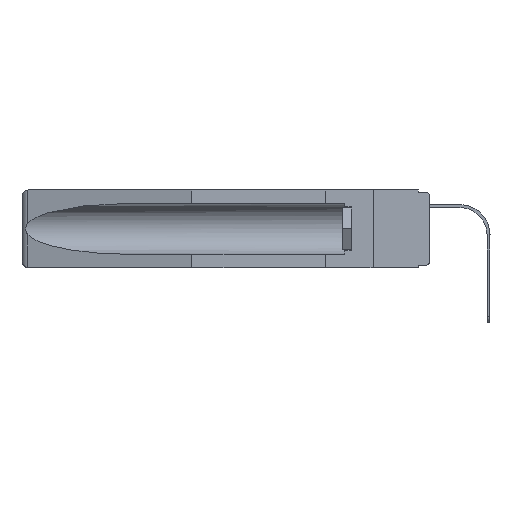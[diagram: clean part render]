
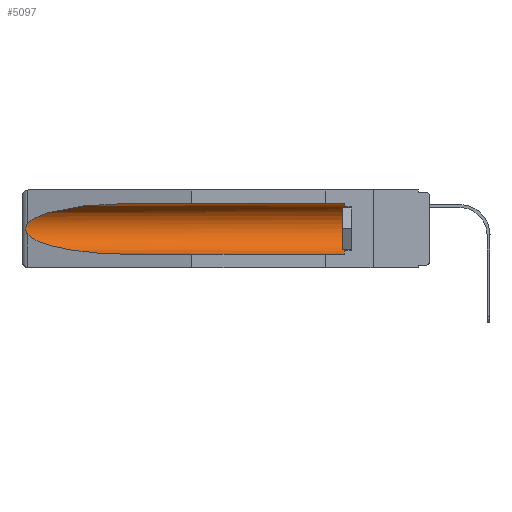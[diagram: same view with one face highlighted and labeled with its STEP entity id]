
A CAD part, left-side view. The second image highlights one B-rep face of the part: STEP entity #5097.
In plain terms, the highlighted cylindrical face has radius 2.857 mm (diameter 5.715 mm), a partial arc.
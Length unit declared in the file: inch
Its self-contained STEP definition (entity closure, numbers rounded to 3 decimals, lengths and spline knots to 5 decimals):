
#67 = DIRECTION ( 'NONE',  ( 0., 1., 0. ) ) ;
#165 = CARTESIAN_POINT ( 'NONE',  ( 0.26597, 1.52961, -0.15275 ) ) ;
#530 = CARTESIAN_POINT ( 'NONE',  ( 0.25451, 1.48313, -0.09465 ) ) ;
#662 = VECTOR ( 'NONE', #4055, 39.37008 ) ;
#757 = ORIENTED_EDGE ( 'NONE', *, *, #12071, .T. ) ;
#1801 = ORIENTED_EDGE ( 'NONE', *, *, #16183, .F. ) ;
#1830 = ORIENTED_EDGE ( 'NONE', *, *, #23367, .T. ) ;
#2187 = VERTEX_POINT ( 'NONE', #19044 ) ;
#2232 = CARTESIAN_POINT ( 'NONE',  ( 0.26597, 1.5296, -0.19026 ) ) ;
#2586 = CARTESIAN_POINT ( 'NONE',  ( 0.21114, 1.30732, -0.284 ) ) ;
#3314 = CARTESIAN_POINT ( 'NONE',  ( 0.26537, 1.52718, -0.19328 ) ) ;
#4028 = CARTESIAN_POINT ( 'NONE',  ( 0.2675, 1.53308, -0.17534 ) ) ;
#4055 = DIRECTION ( 'NONE',  ( 0., 1., 0. ) ) ;
#4277 = DIRECTION ( 'NONE',  ( 0., 1., 0. ) ) ;
#4569 = VERTEX_POINT ( 'NONE', #6419 ) ;
#5097 = ADVANCED_FACE ( 'NONE', ( #5393 ), #23524, .F. ) ;
#5351 = EDGE_CURVE ( 'NONE', #21001, #17451, #7687, .T. ) ;
#5393 = FACE_OUTER_BOUND ( 'NONE', #22505, .T. ) ;
#5844 = CARTESIAN_POINT ( 'NONE',  ( 0.2673, 1.5327, -0.16383 ) ) ;
#6088 = CARTESIAN_POINT ( 'NONE',  ( 0.155, 1.07973, -0.284 ) ) ;
#6222 = CARTESIAN_POINT ( 'NONE',  ( 0.155, 0.126, -0.1715 ) ) ;
#6419 = CARTESIAN_POINT ( 'NONE',  ( 0.26537, 1.52718, -0.14972 ) ) ;
#6507 = VERTEX_POINT ( 'NONE', #9160 ) ;
#6937 = B_SPLINE_CURVE_WITH_KNOTS ( 'NONE', 3,
 ( #16836, #165, #11409, #5844, #13349, #4028, #17066, #18889, #2232, #7668 ),
 .UNSPECIFIED., .F., .F.,
 ( 4, 2, 2, 2, 4 ),
 ( 0., 0.00029, 0.00058, 0.00087, 0.00117 ),
 .UNSPECIFIED. ) ;
#6989 = EDGE_CURVE ( 'NONE', #4569, #21745, #6937, .T. ) ;
#7668 = CARTESIAN_POINT ( 'NONE',  ( 0.26537, 1.52718, -0.19328 ) ) ;
#7679 = CARTESIAN_POINT ( 'NONE',  ( 0.155, -0.30754, -0.284 ) ) ;
#7687 = LINE ( 'NONE', #22410, #662 ) ;
#8291 = ORIENTED_EDGE ( 'NONE', *, *, #6989, .T. ) ;
#9029 = DIRECTION ( 'NONE',  ( 0., 0., 1. ) ) ;
#9063 = VECTOR ( 'NONE', #4277, 39.37008 ) ;
#9160 = CARTESIAN_POINT ( 'NONE',  ( 0.155, 0.126, -0.284 ) ) ;
#9381 = LINE ( 'NONE', #7679, #9063 ) ;
#9707 =( BOUNDED_CURVE ( )  B_SPLINE_CURVE ( 3, ( #17326, #11786, #530, #15147 ),
 .UNSPECIFIED., .F., .F. ) 
 B_SPLINE_CURVE_WITH_KNOTS ( ( 4, 4 ),
 ( 4.71239, 6.08839 ),
 .UNSPECIFIED. ) 
 CURVE ( )  GEOMETRIC_REPRESENTATION_ITEM ( )  RATIONAL_B_SPLINE_CURVE ( ( 1., 0.848, 0.848, 1. ) ) 
 REPRESENTATION_ITEM ( '' )  );
#11300 = DIRECTION ( 'NONE',  ( 0., -1., 0. ) ) ;
#11409 = CARTESIAN_POINT ( 'NONE',  ( 0.26654, 1.53092, -0.15636 ) ) ;
#11769 = CARTESIAN_POINT ( 'NONE',  ( 0.26537, 1.52718, -0.19328 ) ) ;
#11786 = CARTESIAN_POINT ( 'NONE',  ( 0.21114, 1.30732, -0.059 ) ) ;
#12071 = EDGE_CURVE ( 'NONE', #6507, #21001, #17525, .T. ) ;
#12740 = CARTESIAN_POINT ( 'NONE',  ( 0.155, 1.07973, -0.059 ) ) ;
#13182 = EDGE_CURVE ( 'NONE', #17451, #4569, #9707, .T. ) ;
#13349 = CARTESIAN_POINT ( 'NONE',  ( 0.2675, 1.53308, -0.16763 ) ) ;
#13407 = AXIS2_PLACEMENT_3D ( 'NONE', #20119, #67, #9029 ) ;
#14631 =( BOUNDED_CURVE ( )  B_SPLINE_CURVE ( 3, ( #11769, #21182, #2586, #6088 ),
 .UNSPECIFIED., .F., .F. ) 
 B_SPLINE_CURVE_WITH_KNOTS ( ( 4, 4 ),
 ( 0.1948, 1.5708 ),
 .UNSPECIFIED. ) 
 CURVE ( )  GEOMETRIC_REPRESENTATION_ITEM ( )  RATIONAL_B_SPLINE_CURVE ( ( 1., 0.848, 0.848, 1. ) ) 
 REPRESENTATION_ITEM ( '' )  );
#14954 = CARTESIAN_POINT ( 'NONE',  ( 0.155, 0.126, -0.059 ) ) ;
#15147 = CARTESIAN_POINT ( 'NONE',  ( 0.26537, 1.52718, -0.14972 ) ) ;
#15286 = DIRECTION ( 'NONE',  ( 0., 0., 1. ) ) ;
#15632 = ORIENTED_EDGE ( 'NONE', *, *, #13182, .T. ) ;
#16183 = EDGE_CURVE ( 'NONE', #6507, #2187, #9381, .T. ) ;
#16764 = ORIENTED_EDGE ( 'NONE', *, *, #5351, .T. ) ;
#16836 = CARTESIAN_POINT ( 'NONE',  ( 0.26537, 1.52718, -0.14972 ) ) ;
#17066 = CARTESIAN_POINT ( 'NONE',  ( 0.2673, 1.53269, -0.17917 ) ) ;
#17326 = CARTESIAN_POINT ( 'NONE',  ( 0.155, 1.07973, -0.059 ) ) ;
#17451 = VERTEX_POINT ( 'NONE', #12740 ) ;
#17525 = CIRCLE ( 'NONE', #23326, 0.1125 ) ;
#18889 = CARTESIAN_POINT ( 'NONE',  ( 0.26655, 1.53094, -0.18657 ) ) ;
#19044 = CARTESIAN_POINT ( 'NONE',  ( 0.155, 1.07973, -0.284 ) ) ;
#20119 = CARTESIAN_POINT ( 'NONE',  ( 0.155, -0.30754, -0.1715 ) ) ;
#21001 = VERTEX_POINT ( 'NONE', #14954 ) ;
#21182 = CARTESIAN_POINT ( 'NONE',  ( 0.25451, 1.48313, -0.24835 ) ) ;
#21745 = VERTEX_POINT ( 'NONE', #3314 ) ;
#22410 = CARTESIAN_POINT ( 'NONE',  ( 0.155, -0.30754, -0.059 ) ) ;
#22505 = EDGE_LOOP ( 'NONE', ( #15632, #8291, #1830, #1801, #757, #16764 ) ) ;
#23326 = AXIS2_PLACEMENT_3D ( 'NONE', #6222, #11300, #15286 ) ;
#23367 = EDGE_CURVE ( 'NONE', #21745, #2187, #14631, .T. ) ;
#23524 = CYLINDRICAL_SURFACE ( 'NONE', #13407, 0.1125 ) ;
